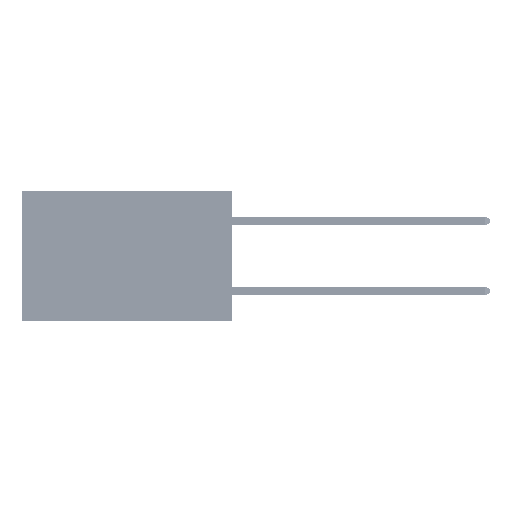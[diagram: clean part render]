
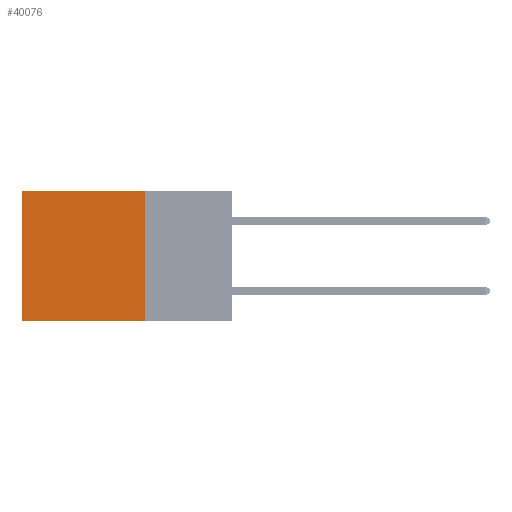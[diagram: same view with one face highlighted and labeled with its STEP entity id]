
A CAD part, left-side view. The second image highlights one B-rep face of the part: STEP entity #40076.
In plain terms, the highlighted planar face has unit normal (-1, 0, 0).
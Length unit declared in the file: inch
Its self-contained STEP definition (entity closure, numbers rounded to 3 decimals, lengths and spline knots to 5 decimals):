
#1919 = EDGE_CURVE ( 'NONE', #44967, #42078, #30075, .T. ) ;
#4202 = DIRECTION ( 'NONE',  ( 0., 0., -1. ) ) ;
#6166 = ORIENTED_EDGE ( 'NONE', *, *, #26854, .T. ) ;
#7115 = DIRECTION ( 'NONE',  ( 0., 1., 0. ) ) ;
#7791 = CARTESIAN_POINT ( 'NONE',  ( 0.2875, 0.25, 0. ) ) ;
#8107 = LINE ( 'NONE', #12262, #48414 ) ;
#9325 = VECTOR ( 'NONE', #7115, 39.37008 ) ;
#11171 = EDGE_CURVE ( 'NONE', #45845, #41824, #17301, .T. ) ;
#12262 = CARTESIAN_POINT ( 'NONE',  ( 0.2875, 0.25, 0. ) ) ;
#13777 = AXIS2_PLACEMENT_3D ( 'NONE', #47750, #43128, #47585 ) ;
#14277 = VECTOR ( 'NONE', #16369, 39.37008 ) ;
#15981 = PLANE ( 'NONE',  #13777 ) ;
#16112 = CARTESIAN_POINT ( 'NONE',  ( 0.2875, 0.25, 0. ) ) ;
#16155 = CARTESIAN_POINT ( 'NONE',  ( 0.2875, 0.6, 0. ) ) ;
#16359 = DIRECTION ( 'NONE',  ( 0., 0., -1. ) ) ;
#16369 = DIRECTION ( 'NONE',  ( 0., 1., 0. ) ) ;
#17301 = LINE ( 'NONE', #35815, #14277 ) ;
#18151 = VECTOR ( 'NONE', #4202, 39.37008 ) ;
#18176 = ORIENTED_EDGE ( 'NONE', *, *, #11171, .F. ) ;
#19477 = EDGE_CURVE ( 'NONE', #44967, #45845, #8107, .T. ) ;
#19711 = ORIENTED_EDGE ( 'NONE', *, *, #19477, .F. ) ;
#21323 = ORIENTED_EDGE ( 'NONE', *, *, #1919, .T. ) ;
#26854 = EDGE_CURVE ( 'NONE', #42078, #41824, #45588, .T. ) ;
#27110 = CARTESIAN_POINT ( 'NONE',  ( 0.2875, 0.6, -0.37 ) ) ;
#27592 = CARTESIAN_POINT ( 'NONE',  ( 0.2875, 0.6, 0. ) ) ;
#30075 = LINE ( 'NONE', #7791, #9325 ) ;
#30534 = CARTESIAN_POINT ( 'NONE',  ( 0.2875, 0.25, -0.37 ) ) ;
#35815 = CARTESIAN_POINT ( 'NONE',  ( 0.2875, 0.25, -0.37 ) ) ;
#36378 = EDGE_LOOP ( 'NONE', ( #6166, #18176, #19711, #21323 ) ) ;
#38145 = FACE_OUTER_BOUND ( 'NONE', #36378, .T. ) ;
#40076 = ADVANCED_FACE ( 'NONE', ( #38145 ), #15981, .F. ) ;
#41824 = VERTEX_POINT ( 'NONE', #27110 ) ;
#42078 = VERTEX_POINT ( 'NONE', #27592 ) ;
#43128 = DIRECTION ( 'NONE',  ( 1., 0., 0. ) ) ;
#44967 = VERTEX_POINT ( 'NONE', #16112 ) ;
#45588 = LINE ( 'NONE', #16155, #18151 ) ;
#45845 = VERTEX_POINT ( 'NONE', #30534 ) ;
#47585 = DIRECTION ( 'NONE',  ( 0., 0., -1. ) ) ;
#47750 = CARTESIAN_POINT ( 'NONE',  ( 0.2875, 0.25, 0. ) ) ;
#48414 = VECTOR ( 'NONE', #16359, 39.37008 ) ;
